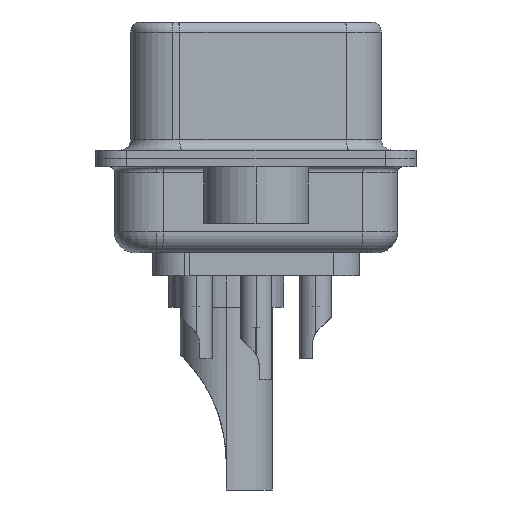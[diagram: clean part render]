
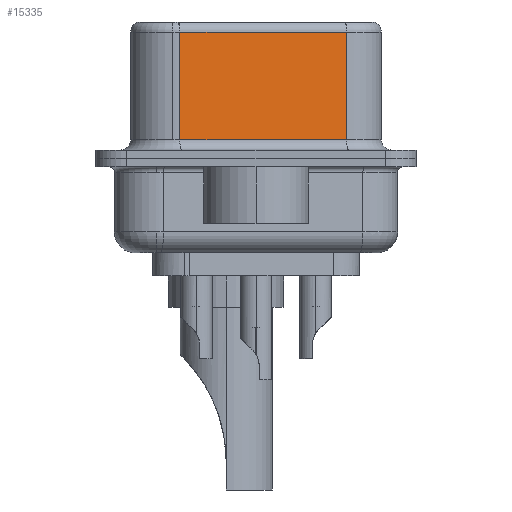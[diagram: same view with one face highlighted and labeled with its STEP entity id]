
A CAD part, left-side view. The second image highlights one B-rep face of the part: STEP entity #15335.
In plain terms, the highlighted planar face has unit normal (-0.985, -0.174, 0).
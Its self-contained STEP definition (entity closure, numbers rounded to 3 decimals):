
#212 = ORIENTED_EDGE ( 'NONE', *, *, #315, .T. ) ;
#315 = EDGE_CURVE ( 'NONE', #26640, #25190, #2889, .T. ) ;
#909 = EDGE_CURVE ( 'NONE', #20342, #4954, #15456, .T. ) ;
#1355 = ORIENTED_EDGE ( 'NONE', *, *, #16580, .T. ) ;
#2208 = EDGE_CURVE ( 'NONE', #25190, #4954, #13320, .T. ) ;
#2889 = LINE ( 'NONE', #16054, #14083 ) ;
#4954 = VERTEX_POINT ( 'NONE', #15741 ) ;
#6491 = DIRECTION ( 'NONE',  ( -0.174, 0.985, 0. ) ) ;
#9403 = CARTESIAN_POINT ( 'NONE',  ( 5.132, -4.322, 6.02 ) ) ;
#12143 = VECTOR ( 'NONE', #6491, 1000. ) ;
#12547 = FACE_OUTER_BOUND ( 'NONE', #27227, .T. ) ;
#12681 = CARTESIAN_POINT ( 'NONE',  ( 5.132, -4.322, 6.52 ) ) ;
#13320 = LINE ( 'NONE', #18218, #18496 ) ;
#14083 = VECTOR ( 'NONE', #19566, 1000. ) ;
#14541 = CARTESIAN_POINT ( 'NONE',  ( 3.73, 3.628, 0.9 ) ) ;
#14933 = DIRECTION ( 'NONE',  ( -0.174, 0.985, 0. ) ) ;
#15335 = ADVANCED_FACE ( 'NONE', ( #12547 ), #26110, .F. ) ;
#15423 = ORIENTED_EDGE ( 'NONE', *, *, #2208, .T. ) ;
#15456 = LINE ( 'NONE', #28890, #20695 ) ;
#15741 = CARTESIAN_POINT ( 'NONE',  ( 5.132, -4.322, 0.9 ) ) ;
#15777 = AXIS2_PLACEMENT_3D ( 'NONE', #12681, #28353, #14933 ) ;
#16054 = CARTESIAN_POINT ( 'NONE',  ( 3.73, 3.628, 6.52 ) ) ;
#16580 = EDGE_CURVE ( 'NONE', #20342, #26640, #18036, .T. ) ;
#18036 = LINE ( 'NONE', #28784, #12143 ) ;
#18068 = DIRECTION ( 'NONE',  ( 0.174, -0.985, 0. ) ) ;
#18218 = CARTESIAN_POINT ( 'NONE',  ( 5.132, -4.322, 0.9 ) ) ;
#18495 = ORIENTED_EDGE ( 'NONE', *, *, #909, .F. ) ;
#18496 = VECTOR ( 'NONE', #18068, 1000. ) ;
#19566 = DIRECTION ( 'NONE',  ( 0., 0., -1. ) ) ;
#20342 = VERTEX_POINT ( 'NONE', #9403 ) ;
#20695 = VECTOR ( 'NONE', #28057, 1000. ) ;
#20776 = CARTESIAN_POINT ( 'NONE',  ( 3.73, 3.628, 6.02 ) ) ;
#25190 = VERTEX_POINT ( 'NONE', #14541 ) ;
#26110 = PLANE ( 'NONE',  #15777 ) ;
#26640 = VERTEX_POINT ( 'NONE', #20776 ) ;
#27227 = EDGE_LOOP ( 'NONE', ( #18495, #1355, #212, #15423 ) ) ;
#28057 = DIRECTION ( 'NONE',  ( 0., 0., -1. ) ) ;
#28353 = DIRECTION ( 'NONE',  ( 0.985, 0.174, 0. ) ) ;
#28784 = CARTESIAN_POINT ( 'NONE',  ( 5.132, -4.322, 6.02 ) ) ;
#28890 = CARTESIAN_POINT ( 'NONE',  ( 5.132, -4.322, 6.52 ) ) ;
